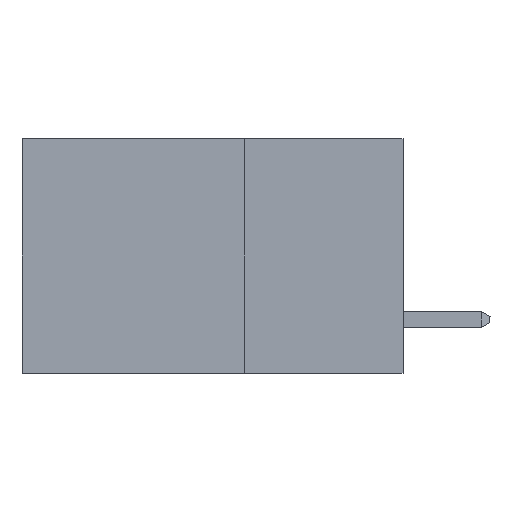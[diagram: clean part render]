
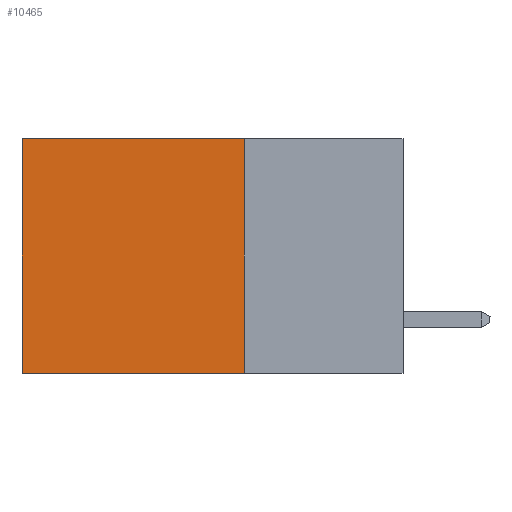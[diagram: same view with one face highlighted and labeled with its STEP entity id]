
A CAD part, left-side view. The second image highlights one B-rep face of the part: STEP entity #10465.
In plain terms, the highlighted planar face has unit normal (-1, 0, 0).
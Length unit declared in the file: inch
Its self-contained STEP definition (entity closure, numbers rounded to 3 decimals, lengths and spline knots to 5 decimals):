
#459 = CARTESIAN_POINT ( 'NONE',  ( 0.2875, 0.25, 0. ) ) ;
#797 = CARTESIAN_POINT ( 'NONE',  ( 0.2875, 0.25, 0. ) ) ;
#1314 = DIRECTION ( 'NONE',  ( 0., 1., 0. ) ) ;
#2895 = AXIS2_PLACEMENT_3D ( 'NONE', #16842, #9264, #4501 ) ;
#3462 = CARTESIAN_POINT ( 'NONE',  ( 0.2875, 0.6, 0. ) ) ;
#4247 = ORIENTED_EDGE ( 'NONE', *, *, #4827, .T. ) ;
#4313 = EDGE_CURVE ( 'NONE', #9511, #7627, #17496, .T. ) ;
#4501 = DIRECTION ( 'NONE',  ( 0., 0., -1. ) ) ;
#4582 = LINE ( 'NONE', #11944, #18661 ) ;
#4827 = EDGE_CURVE ( 'NONE', #9511, #5668, #11774, .T. ) ;
#5668 = VERTEX_POINT ( 'NONE', #11041 ) ;
#6130 = ORIENTED_EDGE ( 'NONE', *, *, #4313, .F. ) ;
#6696 = EDGE_CURVE ( 'NONE', #7627, #14683, #4582, .T. ) ;
#7195 = DIRECTION ( 'NONE',  ( 0., 1., 0. ) ) ;
#7209 = EDGE_CURVE ( 'NONE', #5668, #14683, #9229, .T. ) ;
#7396 = ORIENTED_EDGE ( 'NONE', *, *, #6696, .F. ) ;
#7580 = PLANE ( 'NONE',  #2895 ) ;
#7627 = VERTEX_POINT ( 'NONE', #8314 ) ;
#7941 = DIRECTION ( 'NONE',  ( 0., 0., -1. ) ) ;
#8314 = CARTESIAN_POINT ( 'NONE',  ( 0.2875, 0.25, -0.37 ) ) ;
#9229 = LINE ( 'NONE', #3462, #13239 ) ;
#9264 = DIRECTION ( 'NONE',  ( 1., 0., 0. ) ) ;
#9511 = VERTEX_POINT ( 'NONE', #797 ) ;
#10413 = VECTOR ( 'NONE', #17186, 39.37008 ) ;
#10465 = ADVANCED_FACE ( 'NONE', ( #10854 ), #7580, .F. ) ;
#10854 = FACE_OUTER_BOUND ( 'NONE', #19657, .T. ) ;
#11041 = CARTESIAN_POINT ( 'NONE',  ( 0.2875, 0.6, 0. ) ) ;
#11774 = LINE ( 'NONE', #12988, #19361 ) ;
#11944 = CARTESIAN_POINT ( 'NONE',  ( 0.2875, 0.25, -0.37 ) ) ;
#12988 = CARTESIAN_POINT ( 'NONE',  ( 0.2875, 0.25, 0. ) ) ;
#13239 = VECTOR ( 'NONE', #7941, 39.37008 ) ;
#14683 = VERTEX_POINT ( 'NONE', #15151 ) ;
#15151 = CARTESIAN_POINT ( 'NONE',  ( 0.2875, 0.6, -0.37 ) ) ;
#16474 = ORIENTED_EDGE ( 'NONE', *, *, #7209, .T. ) ;
#16842 = CARTESIAN_POINT ( 'NONE',  ( 0.2875, 0.25, 0. ) ) ;
#17186 = DIRECTION ( 'NONE',  ( 0., 0., -1. ) ) ;
#17496 = LINE ( 'NONE', #459, #10413 ) ;
#18661 = VECTOR ( 'NONE', #1314, 39.37008 ) ;
#19361 = VECTOR ( 'NONE', #7195, 39.37008 ) ;
#19657 = EDGE_LOOP ( 'NONE', ( #16474, #7396, #6130, #4247 ) ) ;
